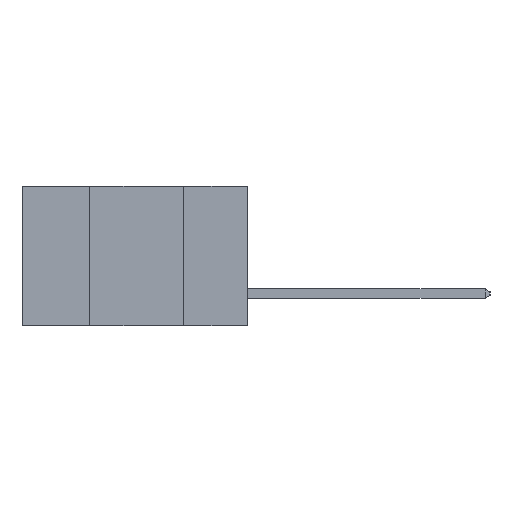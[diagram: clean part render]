
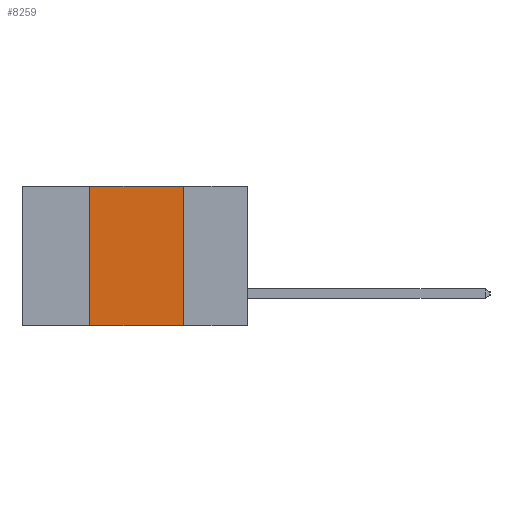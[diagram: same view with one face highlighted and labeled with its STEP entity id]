
A CAD part, left-side view. The second image highlights one B-rep face of the part: STEP entity #8259.
In plain terms, the highlighted planar face has unit normal (-1, 0, 0).
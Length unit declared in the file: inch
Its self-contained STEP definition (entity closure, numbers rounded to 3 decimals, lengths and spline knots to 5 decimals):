
#109 = VECTOR ( 'NONE', #1357, 39.37008 ) ;
#192 = CARTESIAN_POINT ( 'NONE',  ( 0., 0.17, -0.37 ) ) ;
#193 = VERTEX_POINT ( 'NONE', #1567 ) ;
#1357 = DIRECTION ( 'NONE',  ( 0., -1., 0. ) ) ;
#1407 = CARTESIAN_POINT ( 'NONE',  ( 0., 0.6, 0. ) ) ;
#1567 = CARTESIAN_POINT ( 'NONE',  ( 0., 0.42, 0. ) ) ;
#2121 = DIRECTION ( 'NONE',  ( 0., 0., 1. ) ) ;
#2238 = VERTEX_POINT ( 'NONE', #16051 ) ;
#3391 = CARTESIAN_POINT ( 'NONE',  ( 0., 0.17, -0.37 ) ) ;
#3830 = LINE ( 'NONE', #12622, #12127 ) ;
#4144 = EDGE_LOOP ( 'NONE', ( #14575, #20094, #4149, #6490 ) ) ;
#4149 = ORIENTED_EDGE ( 'NONE', *, *, #9780, .F. ) ;
#4561 = EDGE_CURVE ( 'NONE', #193, #16931, #9506, .T. ) ;
#6079 = DIRECTION ( 'NONE',  ( 0., 0., -1. ) ) ;
#6086 = DIRECTION ( 'NONE',  ( 1., 0., 0. ) ) ;
#6107 = CARTESIAN_POINT ( 'NONE',  ( 0., 0.6, 0. ) ) ;
#6234 = PLANE ( 'NONE',  #9548 ) ;
#6490 = ORIENTED_EDGE ( 'NONE', *, *, #12144, .T. ) ;
#6823 = EDGE_CURVE ( 'NONE', #16931, #10147, #14681, .T. ) ;
#7303 = LINE ( 'NONE', #18667, #12015 ) ;
#8259 = ADVANCED_FACE ( 'NONE', ( #11912 ), #6234, .F. ) ;
#9506 = LINE ( 'NONE', #1407, #109 ) ;
#9548 = AXIS2_PLACEMENT_3D ( 'NONE', #6107, #6086, #6079 ) ;
#9780 = EDGE_CURVE ( 'NONE', #2238, #193, #3830, .T. ) ;
#10055 = VECTOR ( 'NONE', #22328, 39.37008 ) ;
#10147 = VERTEX_POINT ( 'NONE', #3391 ) ;
#11912 = FACE_OUTER_BOUND ( 'NONE', #4144, .T. ) ;
#12015 = VECTOR ( 'NONE', #18644, 39.37008 ) ;
#12127 = VECTOR ( 'NONE', #2121, 39.37008 ) ;
#12144 = EDGE_CURVE ( 'NONE', #2238, #10147, #7303, .T. ) ;
#12622 = CARTESIAN_POINT ( 'NONE',  ( 0., 0.42, -0.37 ) ) ;
#14575 = ORIENTED_EDGE ( 'NONE', *, *, #6823, .F. ) ;
#14681 = LINE ( 'NONE', #192, #10055 ) ;
#16051 = CARTESIAN_POINT ( 'NONE',  ( 0., 0.42, -0.37 ) ) ;
#16931 = VERTEX_POINT ( 'NONE', #19288 ) ;
#18644 = DIRECTION ( 'NONE',  ( 0., -1., 0. ) ) ;
#18667 = CARTESIAN_POINT ( 'NONE',  ( 0., 0.6, -0.37 ) ) ;
#19288 = CARTESIAN_POINT ( 'NONE',  ( 0., 0.17, 0. ) ) ;
#20094 = ORIENTED_EDGE ( 'NONE', *, *, #4561, .F. ) ;
#22328 = DIRECTION ( 'NONE',  ( 0., 0., -1. ) ) ;
